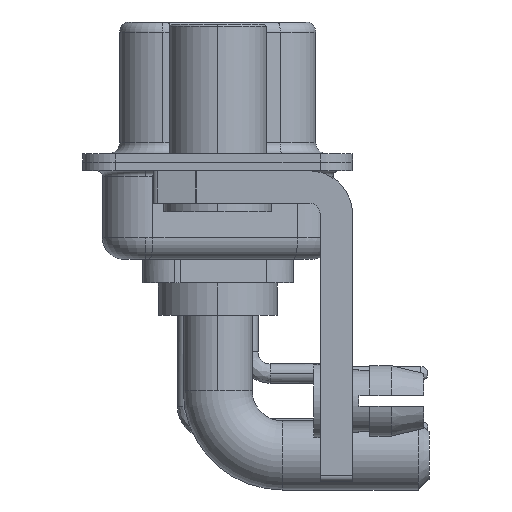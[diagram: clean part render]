
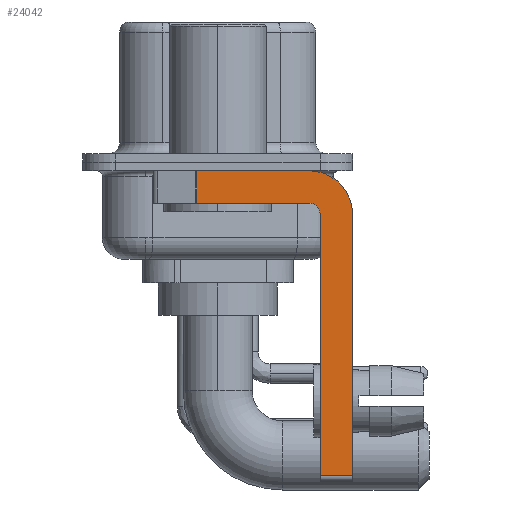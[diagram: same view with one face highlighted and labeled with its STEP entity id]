
A CAD part, left-side view. The second image highlights one B-rep face of the part: STEP entity #24042.
In plain terms, the highlighted planar face has unit normal (-1, 0, 0).
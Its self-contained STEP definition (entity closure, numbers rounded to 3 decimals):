
#27 = EDGE_CURVE ( 'NONE', #3382, #12517, #16862, .T. ) ;
#1454 = CARTESIAN_POINT ( 'NONE',  ( -2.9, -4.25, -2.4 ) ) ;
#1798 = DIRECTION ( 'NONE',  ( 0., 0., 1. ) ) ;
#2889 = CARTESIAN_POINT ( 'NONE',  ( -2.9, -6.25, -2.4 ) ) ;
#3382 = VERTEX_POINT ( 'NONE', #3773 ) ;
#3513 = DIRECTION ( 'NONE',  ( 0., 0., 1. ) ) ;
#3569 = AXIS2_PLACEMENT_3D ( 'NONE', #16441, #8133, #3513 ) ;
#3736 = AXIS2_PLACEMENT_3D ( 'NONE', #6980, #17651, #25762 ) ;
#3773 = CARTESIAN_POINT ( 'NONE',  ( -2.9, -4.75, -14.55 ) ) ;
#3862 = ORIENTED_EDGE ( 'NONE', *, *, #22991, .F. ) ;
#4399 = ORIENTED_EDGE ( 'NONE', *, *, #20655, .F. ) ;
#4730 = LINE ( 'NONE', #21839, #12718 ) ;
#4922 = EDGE_CURVE ( 'NONE', #3382, #22541, #21020, .T. ) ;
#5208 = EDGE_CURVE ( 'NONE', #22585, #7519, #4730, .T. ) ;
#5289 = ORIENTED_EDGE ( 'NONE', *, *, #4922, .F. ) ;
#5531 = DIRECTION ( 'NONE',  ( 1., 0., 0. ) ) ;
#5916 = CARTESIAN_POINT ( 'NONE',  ( -2.9, -4.25, -1.9 ) ) ;
#6102 = CARTESIAN_POINT ( 'NONE',  ( -2.9, -4.75, -2.4 ) ) ;
#6696 = FACE_OUTER_BOUND ( 'NONE', #21581, .T. ) ;
#6826 = VECTOR ( 'NONE', #24410, 1000. ) ;
#6980 = CARTESIAN_POINT ( 'NONE',  ( -2.9, -4.25, -2.4 ) ) ;
#7176 = VERTEX_POINT ( 'NONE', #5916 ) ;
#7329 = LINE ( 'NONE', #15908, #6826 ) ;
#7519 = VERTEX_POINT ( 'NONE', #13797 ) ;
#8133 = DIRECTION ( 'NONE',  ( -1., 0., 0. ) ) ;
#8448 = LINE ( 'NONE', #8581, #22711 ) ;
#8581 = CARTESIAN_POINT ( 'NONE',  ( -2.9, 3., -0.4 ) ) ;
#10387 = DIRECTION ( 'NONE',  ( 0., -1., 0. ) ) ;
#10431 = VERTEX_POINT ( 'NONE', #27394 ) ;
#10908 = ORIENTED_EDGE ( 'NONE', *, *, #16577, .F. ) ;
#11723 = VECTOR ( 'NONE', #26437, 1000. ) ;
#12136 = VECTOR ( 'NONE', #10387, 1000. ) ;
#12344 = CARTESIAN_POINT ( 'NONE',  ( -2.9, -6.25, -2.4 ) ) ;
#12517 = VERTEX_POINT ( 'NONE', #13184 ) ;
#12672 = AXIS2_PLACEMENT_3D ( 'NONE', #1454, #5531, #22893 ) ;
#12718 = VECTOR ( 'NONE', #13601, 1000. ) ;
#13184 = CARTESIAN_POINT ( 'NONE',  ( -2.9, -6.25, -14.55 ) ) ;
#13249 = DIRECTION ( 'NONE',  ( 0., -1., 0. ) ) ;
#13464 = PLANE ( 'NONE',  #3736 ) ;
#13601 = DIRECTION ( 'NONE',  ( 0., 0., -1. ) ) ;
#13797 = CARTESIAN_POINT ( 'NONE',  ( -2.9, 0.978, -1.9 ) ) ;
#14424 = CARTESIAN_POINT ( 'NONE',  ( -2.9, 0.978, -0.4 ) ) ;
#14555 = VECTOR ( 'NONE', #1798, 1000. ) ;
#15290 = ORIENTED_EDGE ( 'NONE', *, *, #18482, .F. ) ;
#15686 = LINE ( 'NONE', #2889, #11723 ) ;
#15908 = CARTESIAN_POINT ( 'NONE',  ( -2.9, -4.25, -1.9 ) ) ;
#16441 = CARTESIAN_POINT ( 'NONE',  ( -2.9, -4.25, -2.4 ) ) ;
#16577 = EDGE_CURVE ( 'NONE', #22585, #10431, #8448, .T. ) ;
#16862 = LINE ( 'NONE', #18944, #12136 ) ;
#17570 = CIRCLE ( 'NONE', #12672, 2. ) ;
#17651 = DIRECTION ( 'NONE',  ( 1., 0., 0. ) ) ;
#18353 = CIRCLE ( 'NONE', #3569, 0.5 ) ;
#18482 = EDGE_CURVE ( 'NONE', #22541, #7176, #18353, .T. ) ;
#18944 = CARTESIAN_POINT ( 'NONE',  ( -2.9, -4.25, -14.55 ) ) ;
#19007 = VERTEX_POINT ( 'NONE', #12344 ) ;
#19733 = ORIENTED_EDGE ( 'NONE', *, *, #23279, .F. ) ;
#20655 = EDGE_CURVE ( 'NONE', #19007, #12517, #15686, .T. ) ;
#21020 = LINE ( 'NONE', #27050, #14555 ) ;
#21581 = EDGE_LOOP ( 'NONE', ( #10908, #24549, #19733, #15290, #5289, #21822, #4399, #3862 ) ) ;
#21822 = ORIENTED_EDGE ( 'NONE', *, *, #27, .T. ) ;
#21839 = CARTESIAN_POINT ( 'NONE',  ( -2.9, 0.978, -1.9 ) ) ;
#22541 = VERTEX_POINT ( 'NONE', #6102 ) ;
#22585 = VERTEX_POINT ( 'NONE', #14424 ) ;
#22711 = VECTOR ( 'NONE', #13249, 1000. ) ;
#22893 = DIRECTION ( 'NONE',  ( 0., 0., -1. ) ) ;
#22991 = EDGE_CURVE ( 'NONE', #10431, #19007, #17570, .T. ) ;
#23279 = EDGE_CURVE ( 'NONE', #7176, #7519, #7329, .T. ) ;
#24042 = ADVANCED_FACE ( 'NONE', ( #6696 ), #13464, .F. ) ;
#24410 = DIRECTION ( 'NONE',  ( 0., 1., 0. ) ) ;
#24549 = ORIENTED_EDGE ( 'NONE', *, *, #5208, .T. ) ;
#25762 = DIRECTION ( 'NONE',  ( 0., 0., -1. ) ) ;
#26437 = DIRECTION ( 'NONE',  ( 0., 0., -1. ) ) ;
#27050 = CARTESIAN_POINT ( 'NONE',  ( -2.9, -4.75, -14.8 ) ) ;
#27394 = CARTESIAN_POINT ( 'NONE',  ( -2.9, -4.25, -0.4 ) ) ;
